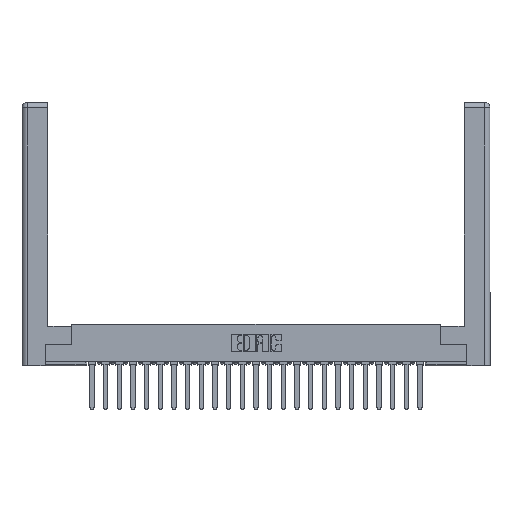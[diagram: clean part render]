
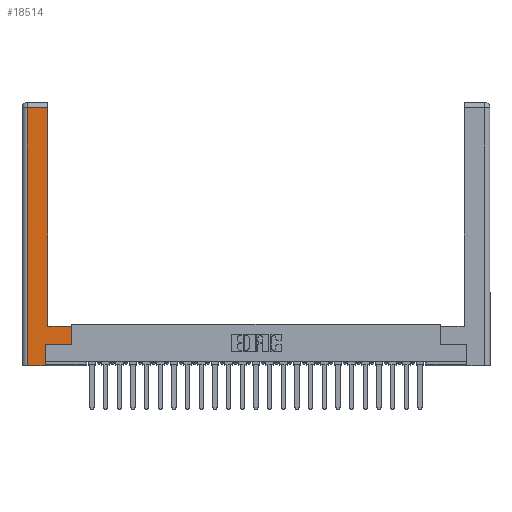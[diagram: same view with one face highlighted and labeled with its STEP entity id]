
A CAD part, top view. The second image highlights one B-rep face of the part: STEP entity #18514.
In plain terms, the highlighted planar face has unit normal (0, 0, 1).
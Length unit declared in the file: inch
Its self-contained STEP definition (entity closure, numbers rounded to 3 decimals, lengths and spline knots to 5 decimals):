
#566 = CARTESIAN_POINT ( 'NONE',  ( 0.565, 0.45, 0. ) ) ;
#617 = CARTESIAN_POINT ( 'NONE',  ( 0.265, 0., 0. ) ) ;
#1020 = EDGE_CURVE ( 'NONE', #11463, #9402, #23254, .T. ) ;
#1046 = LINE ( 'NONE', #19310, #14626 ) ;
#1166 = EDGE_CURVE ( 'NONE', #9988, #19752, #14457, .T. ) ;
#1247 = DIRECTION ( 'NONE',  ( 0., 1., 0. ) ) ;
#1318 = DIRECTION ( 'NONE',  ( 0., 1., 0. ) ) ;
#2191 = CARTESIAN_POINT ( 'NONE',  ( 0., 0., 0. ) ) ;
#3474 = FACE_OUTER_BOUND ( 'NONE', #23786, .T. ) ;
#3622 = ORIENTED_EDGE ( 'NONE', *, *, #19193, .T. ) ;
#3657 = CARTESIAN_POINT ( 'NONE',  ( 0.0615, 2.94, 0. ) ) ;
#4020 = PLANE ( 'NONE',  #14426 ) ;
#4031 = ORIENTED_EDGE ( 'NONE', *, *, #11770, .T. ) ;
#4120 = DIRECTION ( 'NONE',  ( -1., 0., 0. ) ) ;
#5076 = VECTOR ( 'NONE', #1318, 39.37008 ) ;
#5416 = ORIENTED_EDGE ( 'NONE', *, *, #1020, .T. ) ;
#5875 = EDGE_CURVE ( 'NONE', #10939, #25050, #9004, .T. ) ;
#6143 = CARTESIAN_POINT ( 'NONE',  ( 0.0615, 0., 0. ) ) ;
#6450 = CARTESIAN_POINT ( 'NONE',  ( 0.265, 0.245, 0. ) ) ;
#7477 = ORIENTED_EDGE ( 'NONE', *, *, #17293, .T. ) ;
#7972 = DIRECTION ( 'NONE',  ( -1., 0., 0. ) ) ;
#7985 = CARTESIAN_POINT ( 'NONE',  ( 0.295, 0.45, 0. ) ) ;
#8133 = VECTOR ( 'NONE', #4120, 39.37008 ) ;
#9004 = LINE ( 'NONE', #11064, #18117 ) ;
#9084 = VERTEX_POINT ( 'NONE', #22762 ) ;
#9402 = VERTEX_POINT ( 'NONE', #15905 ) ;
#9628 = CARTESIAN_POINT ( 'NONE',  ( 0.295, 3., 0. ) ) ;
#9988 = VERTEX_POINT ( 'NONE', #617 ) ;
#10231 = CARTESIAN_POINT ( 'NONE',  ( 0.565, 0.245, 0. ) ) ;
#10743 = LINE ( 'NONE', #7985, #8133 ) ;
#10939 = VERTEX_POINT ( 'NONE', #10231 ) ;
#11064 = CARTESIAN_POINT ( 'NONE',  ( 0.565, 0.45, 0. ) ) ;
#11463 = VERTEX_POINT ( 'NONE', #11826 ) ;
#11770 = EDGE_CURVE ( 'NONE', #17119, #9988, #1046, .T. ) ;
#11826 = CARTESIAN_POINT ( 'NONE',  ( 0.295, 0.45, 0. ) ) ;
#11979 = EDGE_CURVE ( 'NONE', #25050, #11463, #10743, .T. ) ;
#12178 = LINE ( 'NONE', #25193, #23556 ) ;
#13342 = ORIENTED_EDGE ( 'NONE', *, *, #11979, .T. ) ;
#13544 = ORIENTED_EDGE ( 'NONE', *, *, #5875, .T. ) ;
#14422 = ORIENTED_EDGE ( 'NONE', *, *, #23069, .T. ) ;
#14426 = AXIS2_PLACEMENT_3D ( 'NONE', #2191, #18570, #7972 ) ;
#14457 = LINE ( 'NONE', #19917, #24575 ) ;
#14626 = VECTOR ( 'NONE', #21237, 39.37008 ) ;
#15905 = CARTESIAN_POINT ( 'NONE',  ( 0.295, 2.94, 0. ) ) ;
#16195 = VECTOR ( 'NONE', #18975, 39.37008 ) ;
#16893 = CARTESIAN_POINT ( 'NONE',  ( 0.0615, 0., 0. ) ) ;
#17119 = VERTEX_POINT ( 'NONE', #6143 ) ;
#17293 = EDGE_CURVE ( 'NONE', #9084, #17119, #21706, .T. ) ;
#18117 = VECTOR ( 'NONE', #21310, 39.37008 ) ;
#18514 = ADVANCED_FACE ( 'NONE', ( #3474 ), #4020, .F. ) ;
#18570 = DIRECTION ( 'NONE',  ( 0., 0., -1. ) ) ;
#18975 = DIRECTION ( 'NONE',  ( 0., -1., 0. ) ) ;
#19161 = DIRECTION ( 'NONE',  ( 1., 0., 0. ) ) ;
#19193 = EDGE_CURVE ( 'NONE', #19752, #10939, #12178, .T. ) ;
#19310 = CARTESIAN_POINT ( 'NONE',  ( 0.265, 0., 0. ) ) ;
#19752 = VERTEX_POINT ( 'NONE', #6450 ) ;
#19917 = CARTESIAN_POINT ( 'NONE',  ( 0.265, 0.245, 0. ) ) ;
#21237 = DIRECTION ( 'NONE',  ( 1., 0., 0. ) ) ;
#21252 = VECTOR ( 'NONE', #24440, 39.37008 ) ;
#21310 = DIRECTION ( 'NONE',  ( 0., 1., 0. ) ) ;
#21706 = LINE ( 'NONE', #16893, #16195 ) ;
#22762 = CARTESIAN_POINT ( 'NONE',  ( 0.0615, 2.94, 0. ) ) ;
#23069 = EDGE_CURVE ( 'NONE', #9402, #9084, #26799, .T. ) ;
#23254 = LINE ( 'NONE', #9628, #5076 ) ;
#23556 = VECTOR ( 'NONE', #19161, 39.37008 ) ;
#23786 = EDGE_LOOP ( 'NONE', ( #5416, #14422, #7477, #4031, #26711, #3622, #13544, #13342 ) ) ;
#24440 = DIRECTION ( 'NONE',  ( -1., 0., 0. ) ) ;
#24575 = VECTOR ( 'NONE', #1247, 39.37008 ) ;
#25050 = VERTEX_POINT ( 'NONE', #566 ) ;
#25193 = CARTESIAN_POINT ( 'NONE',  ( 0.565, 0.245, 0. ) ) ;
#26711 = ORIENTED_EDGE ( 'NONE', *, *, #1166, .T. ) ;
#26799 = LINE ( 'NONE', #3657, #21252 ) ;
